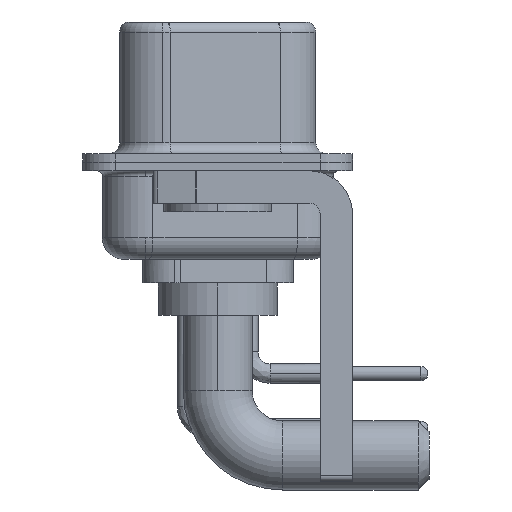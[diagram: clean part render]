
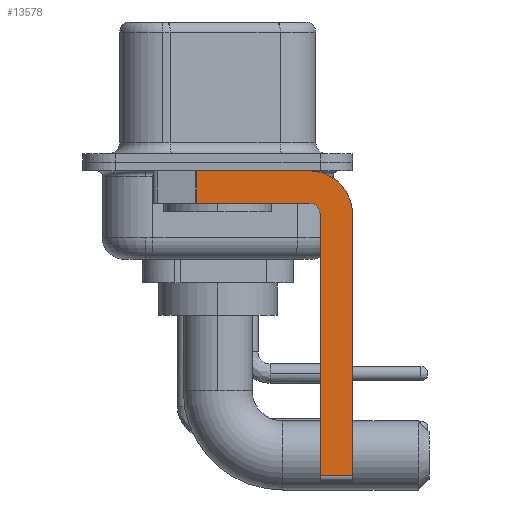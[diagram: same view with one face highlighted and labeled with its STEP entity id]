
A CAD part, left-side view. The second image highlights one B-rep face of the part: STEP entity #13578.
In plain terms, the highlighted planar face has unit normal (-1, 0, 0).
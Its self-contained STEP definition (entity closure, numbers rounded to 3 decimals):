
#173 = EDGE_CURVE ( 'NONE', #12078, #9770, #3152, .T. ) ;
#388 = VERTEX_POINT ( 'NONE', #27375 ) ;
#722 = ORIENTED_EDGE ( 'NONE', *, *, #17469, .F. ) ;
#776 = AXIS2_PLACEMENT_3D ( 'NONE', #10462, #5712, #24837 ) ;
#1274 = VECTOR ( 'NONE', #2417, 1000. ) ;
#1979 = CARTESIAN_POINT ( 'NONE',  ( -2.9, 0.978, -0.4 ) ) ;
#2417 = DIRECTION ( 'NONE',  ( 0., 0., -1. ) ) ;
#3152 = LINE ( 'NONE', #17772, #20012 ) ;
#3443 = CIRCLE ( 'NONE', #776, 0.5 ) ;
#4540 = VERTEX_POINT ( 'NONE', #27361 ) ;
#4746 = ORIENTED_EDGE ( 'NONE', *, *, #12427, .F. ) ;
#4967 = DIRECTION ( 'NONE',  ( 1., 0., 0. ) ) ;
#5515 = EDGE_CURVE ( 'NONE', #27175, #388, #20925, .T. ) ;
#5712 = DIRECTION ( 'NONE',  ( -1., 0., 0. ) ) ;
#5936 = ORIENTED_EDGE ( 'NONE', *, *, #26569, .T. ) ;
#6275 = DIRECTION ( 'NONE',  ( 0., 0., -1. ) ) ;
#6462 = CARTESIAN_POINT ( 'NONE',  ( -2.9, -4.75, -14.8 ) ) ;
#7054 = CARTESIAN_POINT ( 'NONE',  ( -2.9, -4.25, -2.4 ) ) ;
#7589 = DIRECTION ( 'NONE',  ( 0., -1., 0. ) ) ;
#7759 = VECTOR ( 'NONE', #6275, 1000. ) ;
#7986 = VECTOR ( 'NONE', #22604, 1000. ) ;
#8386 = VERTEX_POINT ( 'NONE', #16926 ) ;
#8577 = ORIENTED_EDGE ( 'NONE', *, *, #5515, .F. ) ;
#8618 = DIRECTION ( 'NONE',  ( 0., 0., -1. ) ) ;
#9366 = CARTESIAN_POINT ( 'NONE',  ( -2.9, -4.25, -14.55 ) ) ;
#9729 = CARTESIAN_POINT ( 'NONE',  ( -2.9, -6.25, -2.4 ) ) ;
#9770 = VERTEX_POINT ( 'NONE', #22771 ) ;
#10122 = VERTEX_POINT ( 'NONE', #10899 ) ;
#10263 = ORIENTED_EDGE ( 'NONE', *, *, #26741, .T. ) ;
#10462 = CARTESIAN_POINT ( 'NONE',  ( -2.9, -4.25, -2.4 ) ) ;
#10643 = CARTESIAN_POINT ( 'NONE',  ( -2.9, 0.978, -1.9 ) ) ;
#10899 = CARTESIAN_POINT ( 'NONE',  ( -2.9, -4.75, -2.4 ) ) ;
#11111 = FACE_OUTER_BOUND ( 'NONE', #24684, .T. ) ;
#12078 = VERTEX_POINT ( 'NONE', #1979 ) ;
#12424 = CARTESIAN_POINT ( 'NONE',  ( -2.9, -6.25, -2.4 ) ) ;
#12427 = EDGE_CURVE ( 'NONE', #8386, #10122, #25579, .T. ) ;
#12718 = EDGE_CURVE ( 'NONE', #10122, #14830, #3443, .T. ) ;
#13284 = LINE ( 'NONE', #10643, #1274 ) ;
#13414 = ORIENTED_EDGE ( 'NONE', *, *, #25312, .F. ) ;
#13484 = DIRECTION ( 'NONE',  ( 0., 0., -1. ) ) ;
#13486 = ORIENTED_EDGE ( 'NONE', *, *, #173, .F. ) ;
#13578 = ADVANCED_FACE ( 'NONE', ( #11111 ), #26168, .F. ) ;
#14159 = VECTOR ( 'NONE', #15924, 1000. ) ;
#14564 = VECTOR ( 'NONE', #23635, 1000. ) ;
#14830 = VERTEX_POINT ( 'NONE', #26846 ) ;
#15924 = DIRECTION ( 'NONE',  ( 0., -1., 0. ) ) ;
#16191 = CARTESIAN_POINT ( 'NONE',  ( -2.9, -4.25, -1.9 ) ) ;
#16926 = CARTESIAN_POINT ( 'NONE',  ( -2.9, -4.75, -14.55 ) ) ;
#17268 = DIRECTION ( 'NONE',  ( 1., 0., 0. ) ) ;
#17286 = AXIS2_PLACEMENT_3D ( 'NONE', #7054, #4967, #13484 ) ;
#17469 = EDGE_CURVE ( 'NONE', #14830, #4540, #26514, .T. ) ;
#17772 = CARTESIAN_POINT ( 'NONE',  ( -2.9, 3., -0.4 ) ) ;
#18016 = LINE ( 'NONE', #9366, #14159 ) ;
#18433 = ORIENTED_EDGE ( 'NONE', *, *, #12718, .F. ) ;
#18549 = CIRCLE ( 'NONE', #20340, 2. ) ;
#20012 = VECTOR ( 'NONE', #7589, 1000. ) ;
#20340 = AXIS2_PLACEMENT_3D ( 'NONE', #23297, #17268, #8618 ) ;
#20925 = LINE ( 'NONE', #12424, #7759 ) ;
#22604 = DIRECTION ( 'NONE',  ( 0., 1., 0. ) ) ;
#22771 = CARTESIAN_POINT ( 'NONE',  ( -2.9, -4.25, -0.4 ) ) ;
#23297 = CARTESIAN_POINT ( 'NONE',  ( -2.9, -4.25, -2.4 ) ) ;
#23635 = DIRECTION ( 'NONE',  ( 0., 0., 1. ) ) ;
#24684 = EDGE_LOOP ( 'NONE', ( #13486, #5936, #722, #18433, #4746, #10263, #8577, #13414 ) ) ;
#24837 = DIRECTION ( 'NONE',  ( 0., 0., 1. ) ) ;
#25312 = EDGE_CURVE ( 'NONE', #9770, #27175, #18549, .T. ) ;
#25579 = LINE ( 'NONE', #6462, #14564 ) ;
#26168 = PLANE ( 'NONE',  #17286 ) ;
#26514 = LINE ( 'NONE', #16191, #7986 ) ;
#26569 = EDGE_CURVE ( 'NONE', #12078, #4540, #13284, .T. ) ;
#26741 = EDGE_CURVE ( 'NONE', #8386, #388, #18016, .T. ) ;
#26846 = CARTESIAN_POINT ( 'NONE',  ( -2.9, -4.25, -1.9 ) ) ;
#27175 = VERTEX_POINT ( 'NONE', #9729 ) ;
#27361 = CARTESIAN_POINT ( 'NONE',  ( -2.9, 0.978, -1.9 ) ) ;
#27375 = CARTESIAN_POINT ( 'NONE',  ( -2.9, -6.25, -14.55 ) ) ;
